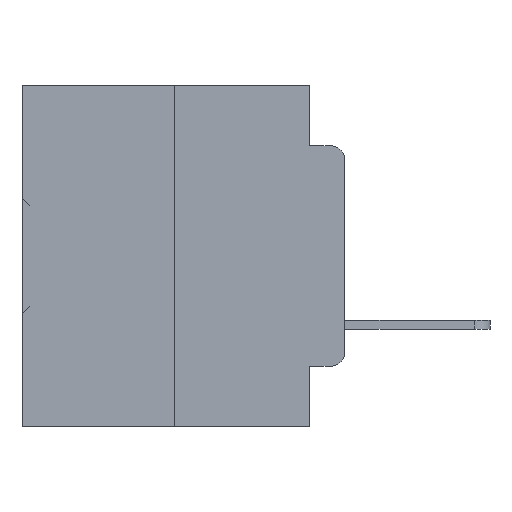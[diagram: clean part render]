
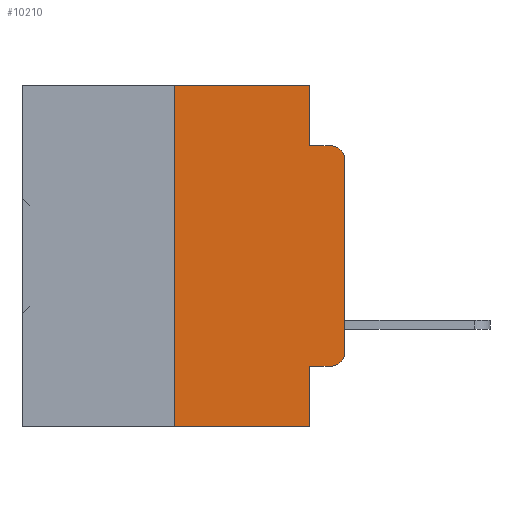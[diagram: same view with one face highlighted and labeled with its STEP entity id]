
A CAD part, left-side view. The second image highlights one B-rep face of the part: STEP entity #10210.
In plain terms, the highlighted planar face has unit normal (-1, 0, 0).
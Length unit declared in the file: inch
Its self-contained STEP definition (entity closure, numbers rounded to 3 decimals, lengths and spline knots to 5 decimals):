
#739 = ORIENTED_EDGE ( 'NONE', *, *, #6026, .T. ) ;
#782 = VERTEX_POINT ( 'NONE', #7619 ) ;
#929 = LINE ( 'NONE', #12189, #8455 ) ;
#1730 = EDGE_CURVE ( 'NONE', #27821, #26135, #34700, .T. ) ;
#2047 = ORIENTED_EDGE ( 'NONE', *, *, #10224, .T. ) ;
#2061 = CARTESIAN_POINT ( 'NONE',  ( 0., 0.25, 0. ) ) ;
#2231 = VECTOR ( 'NONE', #23154, 39.37008 ) ;
#2459 = LINE ( 'NONE', #15730, #25362 ) ;
#2714 = VERTEX_POINT ( 'NONE', #18703 ) ;
#3141 = ORIENTED_EDGE ( 'NONE', *, *, #6809, .F. ) ;
#3142 = DIRECTION ( 'NONE',  ( 0., 0., -1. ) ) ;
#3500 = ORIENTED_EDGE ( 'NONE', *, *, #14985, .F. ) ;
#3586 = ORIENTED_EDGE ( 'NONE', *, *, #30143, .F. ) ;
#4199 = CARTESIAN_POINT ( 'NONE',  ( 0., 0., -0.1085 ) ) ;
#4408 = CIRCLE ( 'NONE', #22551, 0.02 ) ;
#4992 = CIRCLE ( 'NONE', #17437, 0.02 ) ;
#5338 = DIRECTION ( 'NONE',  ( 0., 0., -1. ) ) ;
#5718 = DIRECTION ( 'NONE',  ( 0., 0., -1. ) ) ;
#6026 = EDGE_CURVE ( 'NONE', #25796, #15630, #4992, .T. ) ;
#6143 = LINE ( 'NONE', #22682, #28498 ) ;
#6418 = DIRECTION ( 'NONE',  ( 1., 0., 0. ) ) ;
#6556 = CARTESIAN_POINT ( 'NONE',  ( 0., 0.473, 0. ) ) ;
#6809 = EDGE_CURVE ( 'NONE', #27821, #12358, #12532, .T. ) ;
#7029 = CARTESIAN_POINT ( 'NONE',  ( 0., 0.473, 0. ) ) ;
#7304 = ORIENTED_EDGE ( 'NONE', *, *, #17565, .F. ) ;
#7368 = DIRECTION ( 'NONE',  ( 0., -1., 0. ) ) ;
#7619 = CARTESIAN_POINT ( 'NONE',  ( 0., 0.051, -0.0885 ) ) ;
#8455 = VECTOR ( 'NONE', #34767, 39.37008 ) ;
#8560 = CARTESIAN_POINT ( 'NONE',  ( 0., 0.051, -0.5 ) ) ;
#9169 = CARTESIAN_POINT ( 'NONE',  ( 0., 0.051, -0.4115 ) ) ;
#9515 = VECTOR ( 'NONE', #5338, 39.37008 ) ;
#9681 = PLANE ( 'NONE',  #10966 ) ;
#9767 = ORIENTED_EDGE ( 'NONE', *, *, #1730, .T. ) ;
#10148 = ORIENTED_EDGE ( 'NONE', *, *, #15714, .T. ) ;
#10210 = ADVANCED_FACE ( 'NONE', ( #10865 ), #9681, .F. ) ;
#10224 = EDGE_CURVE ( 'NONE', #23972, #25796, #2459, .T. ) ;
#10865 = FACE_OUTER_BOUND ( 'NONE', #28932, .T. ) ;
#10966 = AXIS2_PLACEMENT_3D ( 'NONE', #6556, #6418, #29806 ) ;
#12189 = CARTESIAN_POINT ( 'NONE',  ( 0., 0.051, -0.0885 ) ) ;
#12358 = VERTEX_POINT ( 'NONE', #35375 ) ;
#12532 = LINE ( 'NONE', #2061, #2231 ) ;
#13173 = VECTOR ( 'NONE', #5718, 39.37008 ) ;
#13823 = DIRECTION ( 'NONE',  ( 0., -1., 0. ) ) ;
#13973 = VECTOR ( 'NONE', #24672, 39.37008 ) ;
#14642 = CARTESIAN_POINT ( 'NONE',  ( 0., 0.02, -0.1085 ) ) ;
#14985 = EDGE_CURVE ( 'NONE', #15216, #782, #21767, .T. ) ;
#15216 = VERTEX_POINT ( 'NONE', #27369 ) ;
#15512 = CARTESIAN_POINT ( 'NONE',  ( 0., 0., -0.3915 ) ) ;
#15630 = VERTEX_POINT ( 'NONE', #29302 ) ;
#15714 = EDGE_CURVE ( 'NONE', #2714, #23972, #4408, .T. ) ;
#15730 = CARTESIAN_POINT ( 'NONE',  ( 0., 0., 0. ) ) ;
#16280 = VERTEX_POINT ( 'NONE', #9169 ) ;
#17437 = AXIS2_PLACEMENT_3D ( 'NONE', #14642, #34247, #17526 ) ;
#17526 = DIRECTION ( 'NONE',  ( 0., 0., -1. ) ) ;
#17565 = EDGE_CURVE ( 'NONE', #12358, #15216, #22562, .T. ) ;
#18503 = CARTESIAN_POINT ( 'NONE',  ( 0., 0.473, -0.5 ) ) ;
#18598 = DIRECTION ( 'NONE',  ( 0., 0., 1. ) ) ;
#18703 = CARTESIAN_POINT ( 'NONE',  ( 0., 0.02, -0.4115 ) ) ;
#21137 = DIRECTION ( 'NONE',  ( -1., 0., 0. ) ) ;
#21767 = LINE ( 'NONE', #34538, #13173 ) ;
#22551 = AXIS2_PLACEMENT_3D ( 'NONE', #37604, #21137, #3142 ) ;
#22562 = LINE ( 'NONE', #7029, #13973 ) ;
#22682 = CARTESIAN_POINT ( 'NONE',  ( 0., 0.051, -0.4115 ) ) ;
#23154 = DIRECTION ( 'NONE',  ( 0., 0., 1. ) ) ;
#23180 = CARTESIAN_POINT ( 'NONE',  ( 0., 0.051, 0. ) ) ;
#23972 = VERTEX_POINT ( 'NONE', #15512 ) ;
#24164 = LINE ( 'NONE', #23180, #9515 ) ;
#24672 = DIRECTION ( 'NONE',  ( 0., -1., 0. ) ) ;
#25362 = VECTOR ( 'NONE', #18598, 39.37008 ) ;
#25796 = VERTEX_POINT ( 'NONE', #4199 ) ;
#26135 = VERTEX_POINT ( 'NONE', #8560 ) ;
#27369 = CARTESIAN_POINT ( 'NONE',  ( 0., 0.051, 0. ) ) ;
#27441 = VECTOR ( 'NONE', #7368, 39.37008 ) ;
#27821 = VERTEX_POINT ( 'NONE', #32308 ) ;
#28498 = VECTOR ( 'NONE', #13823, 39.37008 ) ;
#28932 = EDGE_LOOP ( 'NONE', ( #2047, #739, #3586, #3500, #7304, #3141, #9767, #30450, #30918, #10148 ) ) ;
#29015 = EDGE_CURVE ( 'NONE', #16280, #2714, #6143, .T. ) ;
#29302 = CARTESIAN_POINT ( 'NONE',  ( 0., 0.02, -0.0885 ) ) ;
#29806 = DIRECTION ( 'NONE',  ( 0., 0., -1. ) ) ;
#30143 = EDGE_CURVE ( 'NONE', #782, #15630, #929, .T. ) ;
#30450 = ORIENTED_EDGE ( 'NONE', *, *, #36208, .F. ) ;
#30918 = ORIENTED_EDGE ( 'NONE', *, *, #29015, .T. ) ;
#32308 = CARTESIAN_POINT ( 'NONE',  ( 0., 0.25, -0.5 ) ) ;
#34247 = DIRECTION ( 'NONE',  ( -1., 0., 0. ) ) ;
#34538 = CARTESIAN_POINT ( 'NONE',  ( 0., 0.051, 0. ) ) ;
#34700 = LINE ( 'NONE', #18503, #27441 ) ;
#34767 = DIRECTION ( 'NONE',  ( 0., -1., 0. ) ) ;
#35375 = CARTESIAN_POINT ( 'NONE',  ( 0., 0.25, 0. ) ) ;
#36208 = EDGE_CURVE ( 'NONE', #16280, #26135, #24164, .T. ) ;
#37604 = CARTESIAN_POINT ( 'NONE',  ( 0., 0.02, -0.3915 ) ) ;
